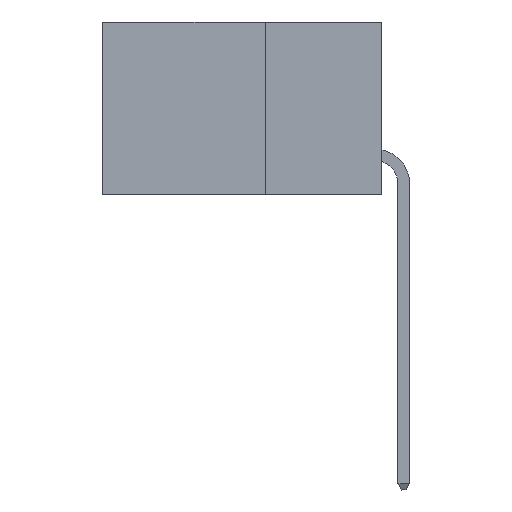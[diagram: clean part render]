
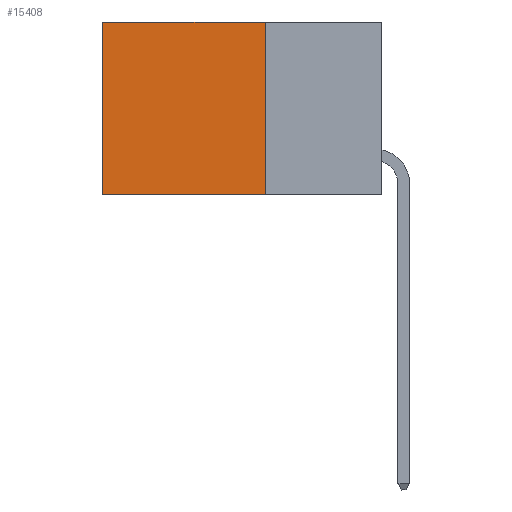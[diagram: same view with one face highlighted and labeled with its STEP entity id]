
A CAD part, left-side view. The second image highlights one B-rep face of the part: STEP entity #15408.
In plain terms, the highlighted planar face has unit normal (-1, 0, 0).
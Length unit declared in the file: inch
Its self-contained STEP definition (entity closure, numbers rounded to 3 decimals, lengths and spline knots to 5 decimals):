
#2242 = VECTOR ( 'NONE', #11705, 39.37008 ) ;
#2278 = AXIS2_PLACEMENT_3D ( 'NONE', #9031, #11484, #4042 ) ;
#2693 = LINE ( 'NONE', #12858, #15869 ) ;
#2794 = EDGE_CURVE ( 'NONE', #6996, #6156, #15499, .T. ) ;
#2848 = CARTESIAN_POINT ( 'NONE',  ( 0.2875, 0.25, 0. ) ) ;
#3689 = LINE ( 'NONE', #2848, #7102 ) ;
#3751 = CARTESIAN_POINT ( 'NONE',  ( 0.2875, 0.25, -0.37 ) ) ;
#4042 = DIRECTION ( 'NONE',  ( 0., 0., -1. ) ) ;
#4338 = ORIENTED_EDGE ( 'NONE', *, *, #15559, .F. ) ;
#5258 = ORIENTED_EDGE ( 'NONE', *, *, #14880, .T. ) ;
#6156 = VERTEX_POINT ( 'NONE', #10799 ) ;
#6722 = VECTOR ( 'NONE', #6904, 39.37008 ) ;
#6904 = DIRECTION ( 'NONE',  ( 0., 1., 0. ) ) ;
#6996 = VERTEX_POINT ( 'NONE', #12337 ) ;
#7102 = VECTOR ( 'NONE', #9157, 39.37008 ) ;
#7606 = VERTEX_POINT ( 'NONE', #8592 ) ;
#7764 = ORIENTED_EDGE ( 'NONE', *, *, #2794, .T. ) ;
#7908 = EDGE_CURVE ( 'NONE', #7606, #13093, #2693, .T. ) ;
#8592 = CARTESIAN_POINT ( 'NONE',  ( 0.2875, 0.25, 0. ) ) ;
#8779 = FACE_OUTER_BOUND ( 'NONE', #9136, .T. ) ;
#9031 = CARTESIAN_POINT ( 'NONE',  ( 0.2875, 0.25, 0. ) ) ;
#9136 = EDGE_LOOP ( 'NONE', ( #7764, #4338, #11227, #5258 ) ) ;
#9157 = DIRECTION ( 'NONE',  ( 0., 1., 0. ) ) ;
#9935 = LINE ( 'NONE', #11745, #6722 ) ;
#10391 = DIRECTION ( 'NONE',  ( 0., 0., -1. ) ) ;
#10794 = CARTESIAN_POINT ( 'NONE',  ( 0.2875, 0.6, 0. ) ) ;
#10799 = CARTESIAN_POINT ( 'NONE',  ( 0.2875, 0.6, -0.37 ) ) ;
#11227 = ORIENTED_EDGE ( 'NONE', *, *, #7908, .F. ) ;
#11484 = DIRECTION ( 'NONE',  ( 1., 0., 0. ) ) ;
#11705 = DIRECTION ( 'NONE',  ( 0., 0., -1. ) ) ;
#11745 = CARTESIAN_POINT ( 'NONE',  ( 0.2875, 0.25, -0.37 ) ) ;
#12337 = CARTESIAN_POINT ( 'NONE',  ( 0.2875, 0.6, 0. ) ) ;
#12858 = CARTESIAN_POINT ( 'NONE',  ( 0.2875, 0.25, 0. ) ) ;
#13093 = VERTEX_POINT ( 'NONE', #3751 ) ;
#14880 = EDGE_CURVE ( 'NONE', #7606, #6996, #3689, .T. ) ;
#15092 = PLANE ( 'NONE',  #2278 ) ;
#15408 = ADVANCED_FACE ( 'NONE', ( #8779 ), #15092, .F. ) ;
#15499 = LINE ( 'NONE', #10794, #2242 ) ;
#15559 = EDGE_CURVE ( 'NONE', #13093, #6156, #9935, .T. ) ;
#15869 = VECTOR ( 'NONE', #10391, 39.37008 ) ;
